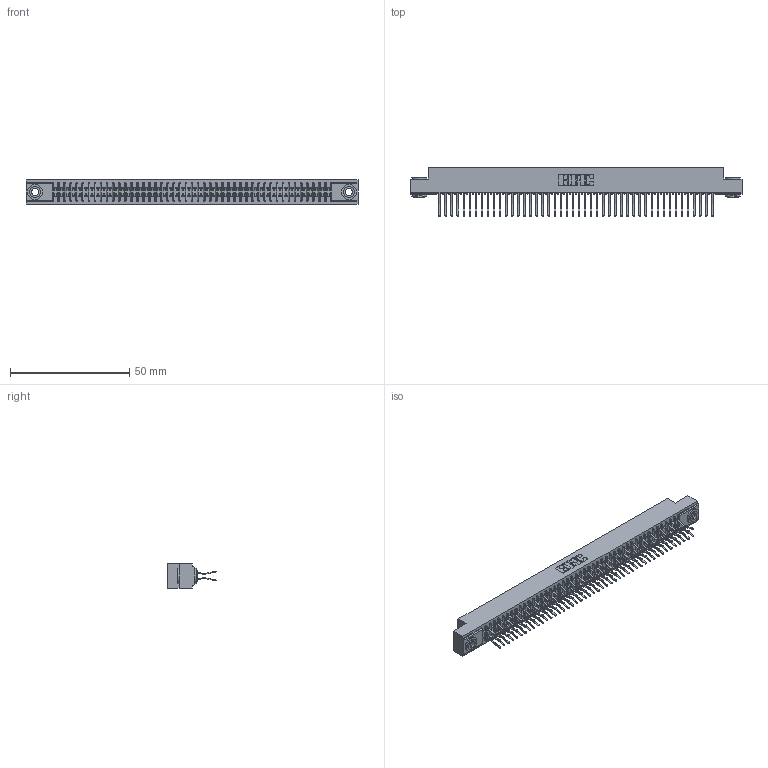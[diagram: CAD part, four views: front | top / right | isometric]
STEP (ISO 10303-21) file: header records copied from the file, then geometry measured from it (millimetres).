
FILE_DESCRIPTION (( 'STEP AP203' ), '1' );
FILE_NAME ('391-092-560-203.STEP', '2018-08-09T18:01:26', ( '' ), ( '' ), 'SwSTEP 2.0', 'SolidWorks 2016', '' );
FILE_SCHEMA (( 'CONFIG_CONTROL_DESIGN' ));
Length unit declared in the file: inch
Products named in the file (4): 341-292-001_341-292-160; 345-250-002_345-250-002-102; 391-092-560-203; 341 Part_.156 (3.96) Dia Mounting Holes
Assembly tree (95 placements, depth 2):
  391-092-560-203
    341 Part_.156 (3.96) Dia Mounting Holes
    341-292-001_341-292-160  x92
    345-250-002_345-250-002-102  x2
Bounding box: 139.06 x 20.37 x 10.16 mm (x, y, z)
Volume: 10365.4 mm3; surface area: 19451.5 mm2
Topology: 95 solids, 95 shells, 6608 faces, 19150 edges, 12422 vertices
Faces by surface type: plane 3772, cylinder 2644, sphere 94, torus 90, cone 8
Entity records: 56342 total; most frequent: CARTESIAN_POINT 9347, ORIENTED_EDGE 9280, DIRECTION 9088, EDGE_CURVE 4640, LINE 3738, VECTOR 3738, VERTEX_POINT 2934, AXIS2_PLACEMENT_3D 2675
